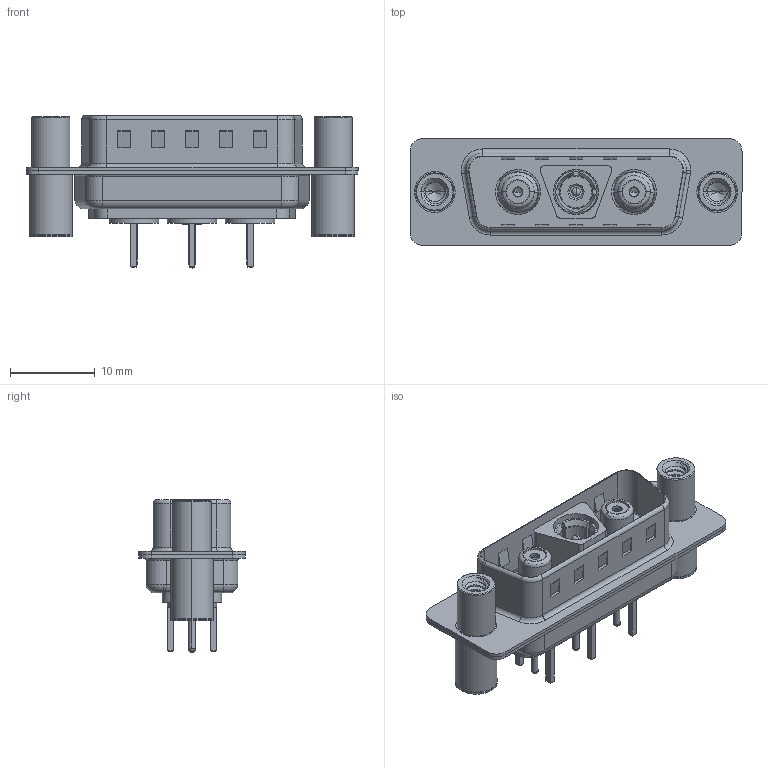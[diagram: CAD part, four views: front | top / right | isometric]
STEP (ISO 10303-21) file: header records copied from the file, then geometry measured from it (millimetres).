
FILE_DESCRIPTION (( 'STEP AP203' ), '1' );
FILE_NAME ('627-3WK3624-5N4.STEP', '2019-06-21T15:49:21', ( '' ), ( '' ), 'SwSTEP 2.0', 'SolidWorks 2016', '' );
FILE_SCHEMA (( 'CONFIG_CONTROL_DESIGN' ));
Length unit declared in the file: millimetre
Products named in the file (15): Insulator Socket 2; Socket_Str; Co-Ax Jack Assy_St; 627Combo Housing_3WK3; 627-3WK3624-5N4; Pin_Str; 627Combo Shell Rear_15 Contacts; Locking Collar; 627Combo Shell Front_15 Contacts; Co-Ax Plug Assy_St; 627Combo Threaded Standoff and Board Spacer_4; Co-Ax Jack_Straight PC Tail; Co-Ax Plug_Straight PC Tail; Insulator Socket; Insulator Pin_Straight PC Tail
Assembly tree (17 placements, depth 3):
  627-3WK3624-5N4
    627Combo Housing_3WK3
    627Combo Shell Rear_15 Contacts
    627Combo Shell Front_15 Contacts
    627Combo Threaded Standoff and Board Spacer_4  x2
    Co-Ax Plug Assy_St
      Co-Ax Plug_Straight PC Tail
      Insulator Pin_Straight PC Tail
      Pin_Str
      Locking Collar
    Co-Ax Jack Assy_St  x2
      Co-Ax Jack_Straight PC Tail
      Insulator Socket
      Insulator Socket 2
      Locking Collar
      Socket_Str
Bounding box: 39.15 x 12.6 x 18 mm (x, y, z)
Volume: 2303 mm3; surface area: 6608.1 mm2
Topology: 19 solids, 19 shells, 785 faces, 1913 edges, 1200 vertices
Faces by surface type: cylinder 329, plane 301, torus 66, cone 63, bspline 18, sphere 8
Entity records: 21326 total; most frequent: CARTESIAN_POINT 5448, DIRECTION 3096, ORIENTED_EDGE 2890, EDGE_CURVE 1445, AXIS2_PLACEMENT_3D 1171, VERTEX_POINT 917, VECTOR 754, LINE 754
